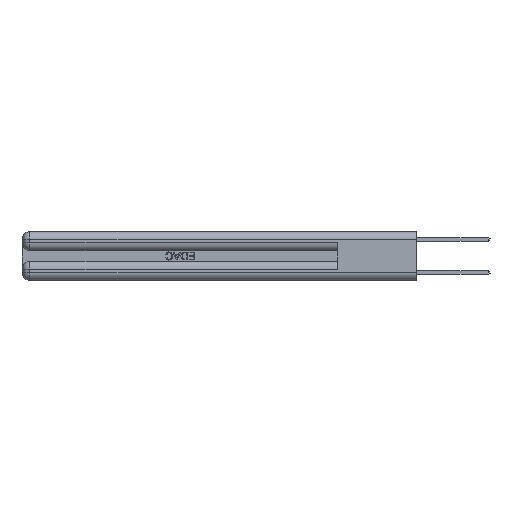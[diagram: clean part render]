
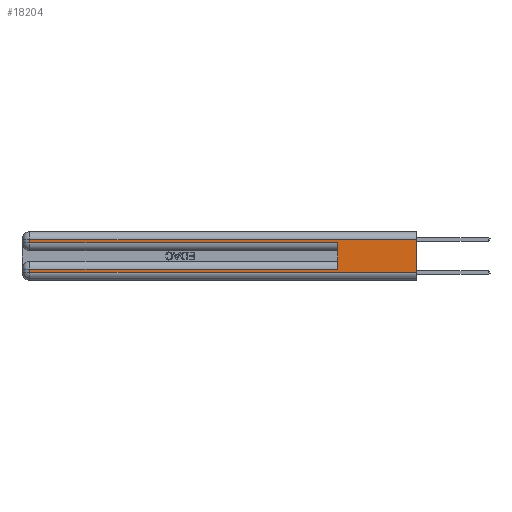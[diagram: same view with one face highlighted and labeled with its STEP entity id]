
A CAD part, left-side view. The second image highlights one B-rep face of the part: STEP entity #18204.
In plain terms, the highlighted planar face has unit normal (-1, 0, 0).
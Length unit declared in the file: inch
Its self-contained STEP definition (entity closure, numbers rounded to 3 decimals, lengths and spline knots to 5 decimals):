
#465 = DIRECTION ( 'NONE',  ( 0., 0., -1. ) ) ;
#654 = ORIENTED_EDGE ( 'NONE', *, *, #29790, .F. ) ;
#702 = CARTESIAN_POINT ( 'NONE',  ( 0., 2.94, 0.06 ) ) ;
#1333 = ORIENTED_EDGE ( 'NONE', *, *, #22108, .T. ) ;
#1423 = ORIENTED_EDGE ( 'NONE', *, *, #26183, .F. ) ;
#3574 = PLANE ( 'NONE',  #8515 ) ;
#3848 = VECTOR ( 'NONE', #28276, 39.37008 ) ;
#4490 = EDGE_CURVE ( 'NONE', #22126, #24530, #8561, .T. ) ;
#4530 = EDGE_CURVE ( 'NONE', #17017, #7409, #28792, .T. ) ;
#4602 = DIRECTION ( 'NONE',  ( 0., -1., 0. ) ) ;
#5342 = CARTESIAN_POINT ( 'NONE',  ( 0., 0., 0.31 ) ) ;
#5846 = VECTOR ( 'NONE', #4602, 39.37008 ) ;
#6227 = CARTESIAN_POINT ( 'NONE',  ( 0., 0., 0.285 ) ) ;
#6800 = CARTESIAN_POINT ( 'NONE',  ( 0., 0., 0.37 ) ) ;
#7409 = VERTEX_POINT ( 'NONE', #17745 ) ;
#7426 = ORIENTED_EDGE ( 'NONE', *, *, #24785, .T. ) ;
#8515 = AXIS2_PLACEMENT_3D ( 'NONE', #6800, #14753, #20166 ) ;
#8561 = LINE ( 'NONE', #27908, #28070 ) ;
#9326 = FACE_OUTER_BOUND ( 'NONE', #10308, .T. ) ;
#10018 = CARTESIAN_POINT ( 'NONE',  ( 0., 0., 0.06 ) ) ;
#10308 = EDGE_LOOP ( 'NONE', ( #654, #1333, #23605, #20237, #1423, #7426, #29732, #33736 ) ) ;
#10496 = VERTEX_POINT ( 'NONE', #33819 ) ;
#10806 = DIRECTION ( 'NONE',  ( 0., 0., 1. ) ) ;
#14753 = DIRECTION ( 'NONE',  ( 1., 0., 0. ) ) ;
#15669 = CARTESIAN_POINT ( 'NONE',  ( 0., 0.6, 0.285 ) ) ;
#16362 = DIRECTION ( 'NONE',  ( 0., 1., 0. ) ) ;
#17017 = VERTEX_POINT ( 'NONE', #27551 ) ;
#17745 = CARTESIAN_POINT ( 'NONE',  ( 0., 2.94, 0.285 ) ) ;
#17933 = VECTOR ( 'NONE', #16362, 39.37008 ) ;
#18204 = ADVANCED_FACE ( 'NONE', ( #9326 ), #3574, .F. ) ;
#18774 = EDGE_CURVE ( 'NONE', #7409, #21934, #19941, .T. ) ;
#19768 = VERTEX_POINT ( 'NONE', #25685 ) ;
#19941 = LINE ( 'NONE', #6227, #3848 ) ;
#20166 = DIRECTION ( 'NONE',  ( 0., 0., -1. ) ) ;
#20237 = ORIENTED_EDGE ( 'NONE', *, *, #18774, .T. ) ;
#20310 = CARTESIAN_POINT ( 'NONE',  ( 0., 0., 0.37 ) ) ;
#20408 = VERTEX_POINT ( 'NONE', #20936 ) ;
#20936 = CARTESIAN_POINT ( 'NONE',  ( 0., 0.6, 0.085 ) ) ;
#21650 = LINE ( 'NONE', #26905, #34868 ) ;
#21934 = VERTEX_POINT ( 'NONE', #15669 ) ;
#22108 = EDGE_CURVE ( 'NONE', #19768, #17017, #24865, .T. ) ;
#22126 = VERTEX_POINT ( 'NONE', #30465 ) ;
#22340 = EDGE_CURVE ( 'NONE', #24530, #10496, #32907, .T. ) ;
#23041 = LINE ( 'NONE', #20310, #29188 ) ;
#23605 = ORIENTED_EDGE ( 'NONE', *, *, #4530, .T. ) ;
#24530 = VERTEX_POINT ( 'NONE', #702 ) ;
#24785 = EDGE_CURVE ( 'NONE', #20408, #22126, #27922, .T. ) ;
#24865 = LINE ( 'NONE', #5342, #17933 ) ;
#25040 = DIRECTION ( 'NONE',  ( 0., 1., 0. ) ) ;
#25685 = CARTESIAN_POINT ( 'NONE',  ( 0., 0., 0.31 ) ) ;
#25717 = CARTESIAN_POINT ( 'NONE',  ( 0., 2.94, 0.37 ) ) ;
#25777 = VECTOR ( 'NONE', #31498, 39.37008 ) ;
#26183 = EDGE_CURVE ( 'NONE', #20408, #21934, #21650, .T. ) ;
#26905 = CARTESIAN_POINT ( 'NONE',  ( 0., 0.6, 0.145 ) ) ;
#27551 = CARTESIAN_POINT ( 'NONE',  ( 0., 2.94, 0.31 ) ) ;
#27908 = CARTESIAN_POINT ( 'NONE',  ( 0., 2.94, 0.37 ) ) ;
#27922 = LINE ( 'NONE', #32628, #29070 ) ;
#28070 = VECTOR ( 'NONE', #465, 39.37008 ) ;
#28276 = DIRECTION ( 'NONE',  ( 0., -1., 0. ) ) ;
#28792 = LINE ( 'NONE', #25717, #25777 ) ;
#29070 = VECTOR ( 'NONE', #25040, 39.37008 ) ;
#29188 = VECTOR ( 'NONE', #34057, 39.37008 ) ;
#29732 = ORIENTED_EDGE ( 'NONE', *, *, #4490, .T. ) ;
#29790 = EDGE_CURVE ( 'NONE', #19768, #10496, #23041, .T. ) ;
#30465 = CARTESIAN_POINT ( 'NONE',  ( 0., 2.94, 0.085 ) ) ;
#31498 = DIRECTION ( 'NONE',  ( 0., 0., -1. ) ) ;
#32628 = CARTESIAN_POINT ( 'NONE',  ( 0., 0., 0.085 ) ) ;
#32907 = LINE ( 'NONE', #10018, #5846 ) ;
#33736 = ORIENTED_EDGE ( 'NONE', *, *, #22340, .T. ) ;
#33819 = CARTESIAN_POINT ( 'NONE',  ( 0., 0., 0.06 ) ) ;
#34057 = DIRECTION ( 'NONE',  ( 0., 0., -1. ) ) ;
#34868 = VECTOR ( 'NONE', #10806, 39.37008 ) ;
